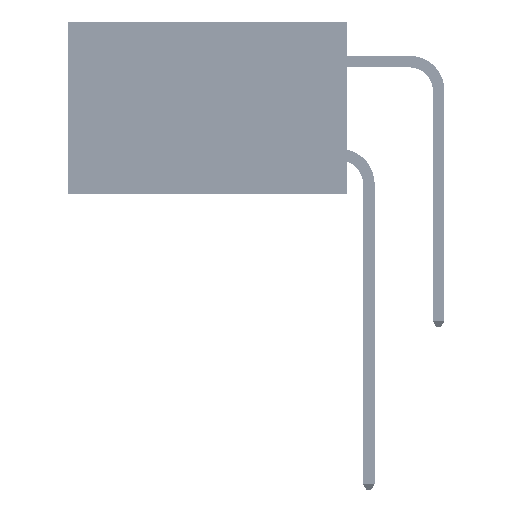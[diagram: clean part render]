
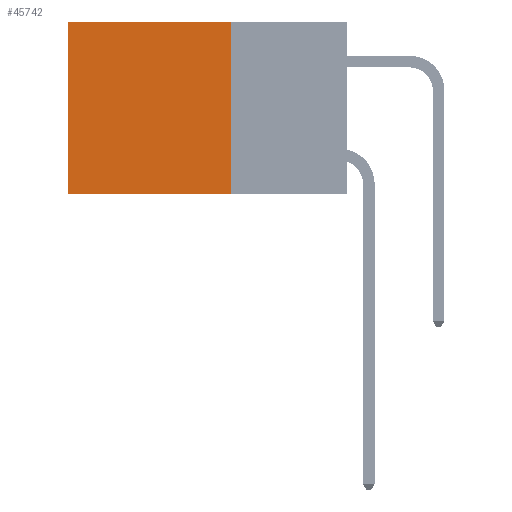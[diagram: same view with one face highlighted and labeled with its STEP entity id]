
A CAD part, left-side view. The second image highlights one B-rep face of the part: STEP entity #45742.
In plain terms, the highlighted planar face has unit normal (-1, 0, 0).
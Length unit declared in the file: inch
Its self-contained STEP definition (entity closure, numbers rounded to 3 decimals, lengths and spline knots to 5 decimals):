
#120 = CARTESIAN_POINT ( 'NONE',  ( 0.2875, 0.25, 0. ) ) ;
#5155 = VECTOR ( 'NONE', #37241, 39.37008 ) ;
#5328 = VERTEX_POINT ( 'NONE', #23457 ) ;
#5780 = EDGE_CURVE ( 'NONE', #19589, #5328, #8178, .T. ) ;
#7781 = ORIENTED_EDGE ( 'NONE', *, *, #5780, .F. ) ;
#8178 = LINE ( 'NONE', #15595, #28053 ) ;
#8713 = VERTEX_POINT ( 'NONE', #10115 ) ;
#9324 = FACE_OUTER_BOUND ( 'NONE', #30101, .T. ) ;
#9395 = CARTESIAN_POINT ( 'NONE',  ( 0.2875, 0.6, -0.37 ) ) ;
#9763 = VERTEX_POINT ( 'NONE', #9395 ) ;
#10115 = CARTESIAN_POINT ( 'NONE',  ( 0.2875, 0.6, 0. ) ) ;
#10609 = EDGE_CURVE ( 'NONE', #5328, #9763, #25343, .T. ) ;
#12735 = ORIENTED_EDGE ( 'NONE', *, *, #13144, .T. ) ;
#13144 = EDGE_CURVE ( 'NONE', #19589, #8713, #24408, .T. ) ;
#14366 = DIRECTION ( 'NONE',  ( 0., 1., 0. ) ) ;
#14928 = DIRECTION ( 'NONE',  ( 1., 0., 0. ) ) ;
#15595 = CARTESIAN_POINT ( 'NONE',  ( 0.2875, 0.25, 0. ) ) ;
#15658 = VECTOR ( 'NONE', #14366, 39.37008 ) ;
#19489 = VECTOR ( 'NONE', #42124, 39.37008 ) ;
#19589 = VERTEX_POINT ( 'NONE', #24141 ) ;
#23457 = CARTESIAN_POINT ( 'NONE',  ( 0.2875, 0.25, -0.37 ) ) ;
#24141 = CARTESIAN_POINT ( 'NONE',  ( 0.2875, 0.25, 0. ) ) ;
#24408 = LINE ( 'NONE', #44172, #5155 ) ;
#25281 = ORIENTED_EDGE ( 'NONE', *, *, #10609, .F. ) ;
#25343 = LINE ( 'NONE', #39566, #15658 ) ;
#26156 = AXIS2_PLACEMENT_3D ( 'NONE', #120, #14928, #40287 ) ;
#27978 = ORIENTED_EDGE ( 'NONE', *, *, #46083, .T. ) ;
#28053 = VECTOR ( 'NONE', #29928, 39.37008 ) ;
#28934 = PLANE ( 'NONE',  #26156 ) ;
#29928 = DIRECTION ( 'NONE',  ( 0., 0., -1. ) ) ;
#30101 = EDGE_LOOP ( 'NONE', ( #27978, #25281, #7781, #12735 ) ) ;
#36526 = LINE ( 'NONE', #38521, #19489 ) ;
#37241 = DIRECTION ( 'NONE',  ( 0., 1., 0. ) ) ;
#38521 = CARTESIAN_POINT ( 'NONE',  ( 0.2875, 0.6, 0. ) ) ;
#39566 = CARTESIAN_POINT ( 'NONE',  ( 0.2875, 0.25, -0.37 ) ) ;
#40287 = DIRECTION ( 'NONE',  ( 0., 0., -1. ) ) ;
#42124 = DIRECTION ( 'NONE',  ( 0., 0., -1. ) ) ;
#44172 = CARTESIAN_POINT ( 'NONE',  ( 0.2875, 0.25, 0. ) ) ;
#45742 = ADVANCED_FACE ( 'NONE', ( #9324 ), #28934, .F. ) ;
#46083 = EDGE_CURVE ( 'NONE', #8713, #9763, #36526, .T. ) ;
